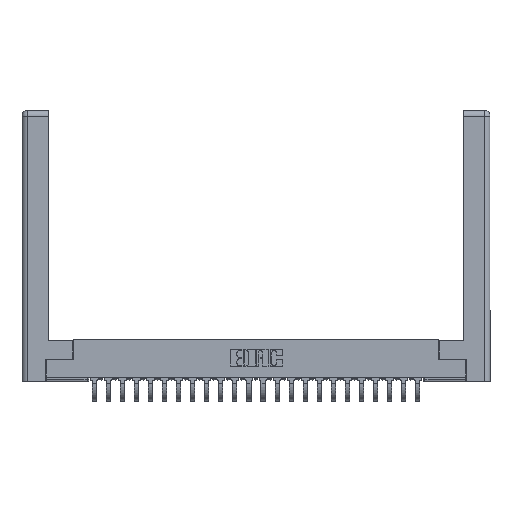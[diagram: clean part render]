
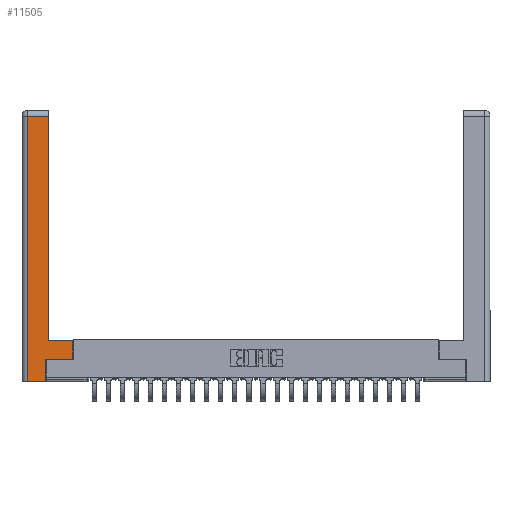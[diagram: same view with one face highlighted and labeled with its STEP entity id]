
A CAD part, top view. The second image highlights one B-rep face of the part: STEP entity #11505.
In plain terms, the highlighted planar face has unit normal (0, 0, 1).
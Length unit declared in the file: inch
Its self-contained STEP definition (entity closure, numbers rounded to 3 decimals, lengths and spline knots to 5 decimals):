
#1328 = CARTESIAN_POINT ( 'NONE',  ( 0.0615, 0., 0. ) ) ;
#1364 = LINE ( 'NONE', #26697, #10175 ) ;
#1822 = VERTEX_POINT ( 'NONE', #18165 ) ;
#1906 = EDGE_CURVE ( 'NONE', #9707, #18924, #1364, .T. ) ;
#1986 = FACE_OUTER_BOUND ( 'NONE', #5045, .T. ) ;
#2126 = LINE ( 'NONE', #6744, #17068 ) ;
#2471 = CARTESIAN_POINT ( 'NONE',  ( 0.295, 0.45, 0. ) ) ;
#2644 = VERTEX_POINT ( 'NONE', #21982 ) ;
#3112 = ORIENTED_EDGE ( 'NONE', *, *, #3629, .T. ) ;
#3380 = EDGE_CURVE ( 'NONE', #21126, #1822, #25146, .T. ) ;
#3629 = EDGE_CURVE ( 'NONE', #1822, #9707, #22467, .T. ) ;
#4051 = LINE ( 'NONE', #12591, #6879 ) ;
#4225 = ORIENTED_EDGE ( 'NONE', *, *, #11471, .T. ) ;
#4303 = CARTESIAN_POINT ( 'NONE',  ( 0.0615, 2.94, 0. ) ) ;
#4656 = DIRECTION ( 'NONE',  ( -1., 0., 0. ) ) ;
#5045 = EDGE_LOOP ( 'NONE', ( #10693, #14544, #3112, #8977, #13456, #6227, #4225, #12894 ) ) ;
#5068 = CARTESIAN_POINT ( 'NONE',  ( 0.295, 0.45, 0. ) ) ;
#5264 = CARTESIAN_POINT ( 'NONE',  ( 0.0615, 0., 0. ) ) ;
#5493 = EDGE_CURVE ( 'NONE', #14738, #21126, #4051, .T. ) ;
#6227 = ORIENTED_EDGE ( 'NONE', *, *, #19591, .T. ) ;
#6654 = CARTESIAN_POINT ( 'NONE',  ( 0.265, 0., 0. ) ) ;
#6744 = CARTESIAN_POINT ( 'NONE',  ( 0.565, 0.45, 0. ) ) ;
#6879 = VECTOR ( 'NONE', #21101, 39.37008 ) ;
#8977 = ORIENTED_EDGE ( 'NONE', *, *, #1906, .T. ) ;
#9289 = LINE ( 'NONE', #5068, #26513 ) ;
#9301 = EDGE_CURVE ( 'NONE', #10378, #14738, #9289, .T. ) ;
#9707 = VERTEX_POINT ( 'NONE', #1328 ) ;
#9845 = CARTESIAN_POINT ( 'NONE',  ( 0.295, 2.94, 0. ) ) ;
#10175 = VECTOR ( 'NONE', #22761, 39.37008 ) ;
#10378 = VERTEX_POINT ( 'NONE', #10968 ) ;
#10684 = CARTESIAN_POINT ( 'NONE',  ( 0., 0., 0. ) ) ;
#10693 = ORIENTED_EDGE ( 'NONE', *, *, #5493, .T. ) ;
#10968 = CARTESIAN_POINT ( 'NONE',  ( 0.565, 0.45, 0. ) ) ;
#11471 = EDGE_CURVE ( 'NONE', #2644, #10378, #2126, .T. ) ;
#11505 = ADVANCED_FACE ( 'NONE', ( #1986 ), #23831, .F. ) ;
#12379 = LINE ( 'NONE', #20888, #17172 ) ;
#12419 = DIRECTION ( 'NONE',  ( -1., 0., 0. ) ) ;
#12591 = CARTESIAN_POINT ( 'NONE',  ( 0.295, 3., 0. ) ) ;
#12894 = ORIENTED_EDGE ( 'NONE', *, *, #9301, .T. ) ;
#13456 = ORIENTED_EDGE ( 'NONE', *, *, #20622, .T. ) ;
#13701 = DIRECTION ( 'NONE',  ( 0., 1., 0. ) ) ;
#14029 = VERTEX_POINT ( 'NONE', #20423 ) ;
#14244 = VECTOR ( 'NONE', #20484, 39.37008 ) ;
#14544 = ORIENTED_EDGE ( 'NONE', *, *, #3380, .T. ) ;
#14738 = VERTEX_POINT ( 'NONE', #2471 ) ;
#15167 = LINE ( 'NONE', #26077, #22912 ) ;
#15290 = DIRECTION ( 'NONE',  ( 0., 1., 0. ) ) ;
#15438 = DIRECTION ( 'NONE',  ( 0., 0., -1. ) ) ;
#17068 = VECTOR ( 'NONE', #15290, 39.37008 ) ;
#17172 = VECTOR ( 'NONE', #13701, 39.37008 ) ;
#18165 = CARTESIAN_POINT ( 'NONE',  ( 0.0615, 2.94, 0. ) ) ;
#18924 = VERTEX_POINT ( 'NONE', #6654 ) ;
#19591 = EDGE_CURVE ( 'NONE', #14029, #2644, #15167, .T. ) ;
#20423 = CARTESIAN_POINT ( 'NONE',  ( 0.265, 0.245, 0. ) ) ;
#20484 = DIRECTION ( 'NONE',  ( 0., -1., 0. ) ) ;
#20616 = AXIS2_PLACEMENT_3D ( 'NONE', #10684, #15438, #25639 ) ;
#20622 = EDGE_CURVE ( 'NONE', #18924, #14029, #12379, .T. ) ;
#20888 = CARTESIAN_POINT ( 'NONE',  ( 0.265, 0.245, 0. ) ) ;
#21101 = DIRECTION ( 'NONE',  ( 0., 1., 0. ) ) ;
#21126 = VERTEX_POINT ( 'NONE', #9845 ) ;
#21732 = VECTOR ( 'NONE', #12419, 39.37008 ) ;
#21982 = CARTESIAN_POINT ( 'NONE',  ( 0.565, 0.245, 0. ) ) ;
#22467 = LINE ( 'NONE', #5264, #14244 ) ;
#22761 = DIRECTION ( 'NONE',  ( 1., 0., 0. ) ) ;
#22912 = VECTOR ( 'NONE', #24268, 39.37008 ) ;
#23831 = PLANE ( 'NONE',  #20616 ) ;
#24268 = DIRECTION ( 'NONE',  ( 1., 0., 0. ) ) ;
#25146 = LINE ( 'NONE', #4303, #21732 ) ;
#25639 = DIRECTION ( 'NONE',  ( -1., 0., 0. ) ) ;
#26077 = CARTESIAN_POINT ( 'NONE',  ( 0.565, 0.245, 0. ) ) ;
#26513 = VECTOR ( 'NONE', #4656, 39.37008 ) ;
#26697 = CARTESIAN_POINT ( 'NONE',  ( 0.265, 0., 0. ) ) ;
